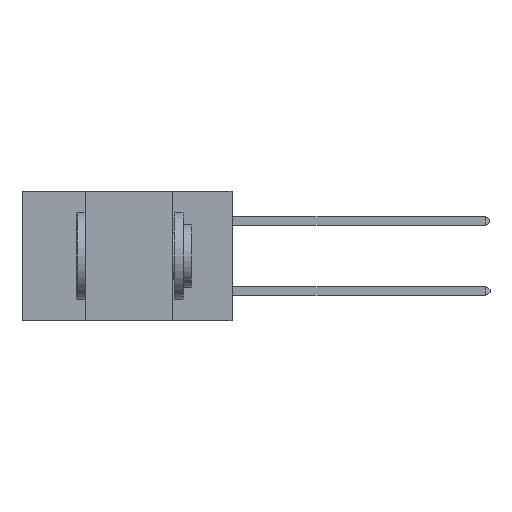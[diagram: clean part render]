
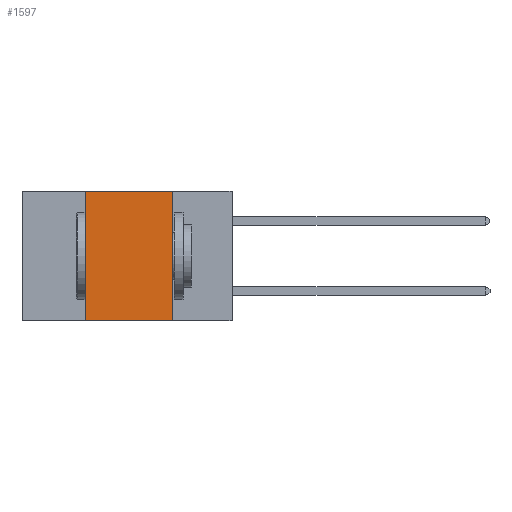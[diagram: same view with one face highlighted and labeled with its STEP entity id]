
A CAD part, left-side view. The second image highlights one B-rep face of the part: STEP entity #1597.
In plain terms, the highlighted planar face has unit normal (-1, 0, 0).
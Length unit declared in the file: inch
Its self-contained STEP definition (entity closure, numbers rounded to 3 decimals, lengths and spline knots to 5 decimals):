
#679 = CARTESIAN_POINT ( 'NONE',  ( 0., 0.17, -0.37 ) ) ;
#1597 = ADVANCED_FACE ( 'NONE', ( #17537 ), #16185, .F. ) ;
#2017 = EDGE_CURVE ( 'NONE', #14471, #5654, #15913, .T. ) ;
#2044 = DIRECTION ( 'NONE',  ( 0., -1., 0. ) ) ;
#2514 = VECTOR ( 'NONE', #4389, 39.37008 ) ;
#2650 = DIRECTION ( 'NONE',  ( 0., -1., 0. ) ) ;
#4201 = VECTOR ( 'NONE', #2650, 39.37008 ) ;
#4210 = CARTESIAN_POINT ( 'NONE',  ( 0., 0.17, 0. ) ) ;
#4282 = VECTOR ( 'NONE', #8011, 39.37008 ) ;
#4389 = DIRECTION ( 'NONE',  ( 0., 0., -1. ) ) ;
#4432 = EDGE_CURVE ( 'NONE', #10559, #5654, #8263, .T. ) ;
#4750 = LINE ( 'NONE', #6272, #4201 ) ;
#5654 = VERTEX_POINT ( 'NONE', #679 ) ;
#5662 = EDGE_CURVE ( 'NONE', #10559, #20282, #9053, .T. ) ;
#6272 = CARTESIAN_POINT ( 'NONE',  ( 0., 0.6, 0. ) ) ;
#7026 = ORIENTED_EDGE ( 'NONE', *, *, #7726, .F. ) ;
#7595 = ORIENTED_EDGE ( 'NONE', *, *, #5662, .F. ) ;
#7719 = VECTOR ( 'NONE', #2044, 39.37008 ) ;
#7726 = EDGE_CURVE ( 'NONE', #20282, #14471, #4750, .T. ) ;
#8011 = DIRECTION ( 'NONE',  ( 0., 0., 1. ) ) ;
#8263 = LINE ( 'NONE', #19404, #7719 ) ;
#9053 = LINE ( 'NONE', #20011, #4282 ) ;
#10559 = VERTEX_POINT ( 'NONE', #19986 ) ;
#14031 = CARTESIAN_POINT ( 'NONE',  ( 0., 0.42, 0. ) ) ;
#14471 = VERTEX_POINT ( 'NONE', #14804 ) ;
#14804 = CARTESIAN_POINT ( 'NONE',  ( 0., 0.17, 0. ) ) ;
#15853 = AXIS2_PLACEMENT_3D ( 'NONE', #16080, #16004, #15927 ) ;
#15913 = LINE ( 'NONE', #4210, #2514 ) ;
#15927 = DIRECTION ( 'NONE',  ( 0., 0., -1. ) ) ;
#16004 = DIRECTION ( 'NONE',  ( 1., 0., 0. ) ) ;
#16080 = CARTESIAN_POINT ( 'NONE',  ( 0., 0.6, 0. ) ) ;
#16185 = PLANE ( 'NONE',  #15853 ) ;
#17537 = FACE_OUTER_BOUND ( 'NONE', #18479, .T. ) ;
#18479 = EDGE_LOOP ( 'NONE', ( #20454, #7026, #7595, #19683 ) ) ;
#19404 = CARTESIAN_POINT ( 'NONE',  ( 0., 0.6, -0.37 ) ) ;
#19683 = ORIENTED_EDGE ( 'NONE', *, *, #4432, .T. ) ;
#19986 = CARTESIAN_POINT ( 'NONE',  ( 0., 0.42, -0.37 ) ) ;
#20011 = CARTESIAN_POINT ( 'NONE',  ( 0., 0.42, 0. ) ) ;
#20282 = VERTEX_POINT ( 'NONE', #14031 ) ;
#20454 = ORIENTED_EDGE ( 'NONE', *, *, #2017, .F. ) ;
